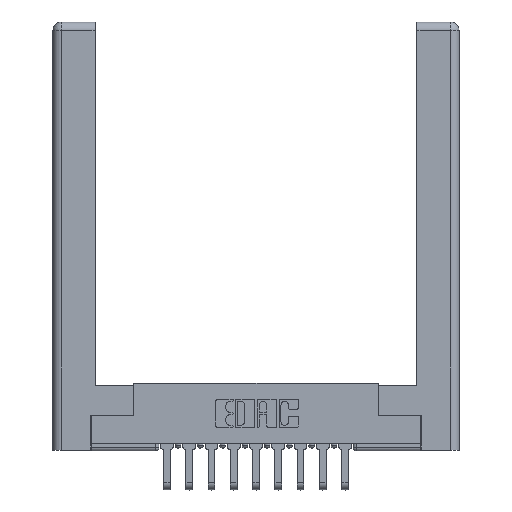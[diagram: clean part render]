
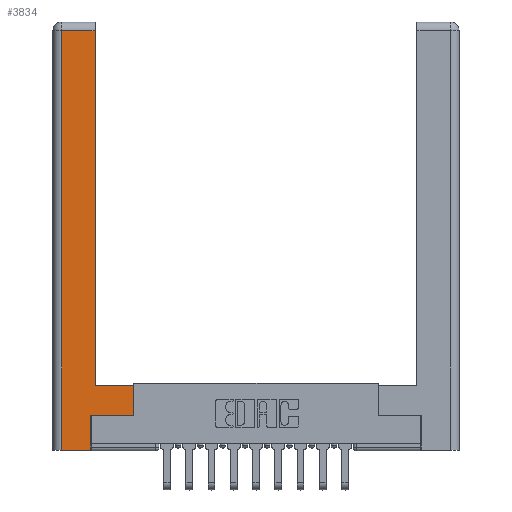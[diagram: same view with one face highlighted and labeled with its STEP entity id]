
A CAD part, top view. The second image highlights one B-rep face of the part: STEP entity #3834.
In plain terms, the highlighted planar face has unit normal (0, 0, 1).
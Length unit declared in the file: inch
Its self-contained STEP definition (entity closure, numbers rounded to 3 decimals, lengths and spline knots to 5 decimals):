
#125 = DIRECTION ( 'NONE',  ( 1., 0., 0. ) ) ;
#744 = CARTESIAN_POINT ( 'NONE',  ( 0.295, 2.94, 0. ) ) ;
#930 = VERTEX_POINT ( 'NONE', #9493 ) ;
#1247 = ORIENTED_EDGE ( 'NONE', *, *, #14229, .T. ) ;
#1302 = CARTESIAN_POINT ( 'NONE',  ( 0.565, 0.45, 0. ) ) ;
#1372 = DIRECTION ( 'NONE',  ( 0., 1., 0. ) ) ;
#1523 = EDGE_CURVE ( 'NONE', #11851, #3310, #7627, .T. ) ;
#1530 = VERTEX_POINT ( 'NONE', #10384 ) ;
#1573 = DIRECTION ( 'NONE',  ( -1., 0., 0. ) ) ;
#1775 = EDGE_CURVE ( 'NONE', #3623, #6599, #8016, .T. ) ;
#1843 = VECTOR ( 'NONE', #1372, 39.37008 ) ;
#1980 = CARTESIAN_POINT ( 'NONE',  ( 0.295, 0.45, 0. ) ) ;
#2111 = LINE ( 'NONE', #1980, #5832 ) ;
#2530 = VECTOR ( 'NONE', #13794, 39.37008 ) ;
#2933 = EDGE_CURVE ( 'NONE', #3310, #3623, #8172, .T. ) ;
#3310 = VERTEX_POINT ( 'NONE', #744 ) ;
#3444 = LINE ( 'NONE', #4160, #3625 ) ;
#3530 = ORIENTED_EDGE ( 'NONE', *, *, #1775, .T. ) ;
#3623 = VERTEX_POINT ( 'NONE', #16143 ) ;
#3625 = VECTOR ( 'NONE', #4552, 39.37008 ) ;
#3834 = ADVANCED_FACE ( 'NONE', ( #15181 ), #9052, .F. ) ;
#4160 = CARTESIAN_POINT ( 'NONE',  ( 0.265, 0., 0. ) ) ;
#4260 = DIRECTION ( 'NONE',  ( -1., 0., 0. ) ) ;
#4552 = DIRECTION ( 'NONE',  ( 1., 0., 0. ) ) ;
#4597 = CARTESIAN_POINT ( 'NONE',  ( 0.0615, 0., 0. ) ) ;
#4900 = LINE ( 'NONE', #6573, #11957 ) ;
#5036 = EDGE_CURVE ( 'NONE', #11642, #930, #8097, .T. ) ;
#5145 = AXIS2_PLACEMENT_3D ( 'NONE', #12853, #15372, #1573 ) ;
#5531 = ORIENTED_EDGE ( 'NONE', *, *, #15434, .T. ) ;
#5742 = VERTEX_POINT ( 'NONE', #1302 ) ;
#5832 = VECTOR ( 'NONE', #4260, 39.37008 ) ;
#6321 = CARTESIAN_POINT ( 'NONE',  ( 0.265, 0.245, 0. ) ) ;
#6382 = EDGE_LOOP ( 'NONE', ( #7853, #10713, #3530, #5531, #9889, #7190, #12267, #1247 ) ) ;
#6568 = CARTESIAN_POINT ( 'NONE',  ( 0.265, 0., 0. ) ) ;
#6573 = CARTESIAN_POINT ( 'NONE',  ( 0.565, 0.45, 0. ) ) ;
#6599 = VERTEX_POINT ( 'NONE', #4597 ) ;
#6864 = CARTESIAN_POINT ( 'NONE',  ( 0.0615, 2.94, 0. ) ) ;
#6979 = EDGE_CURVE ( 'NONE', #1530, #5742, #4900, .T. ) ;
#7190 = ORIENTED_EDGE ( 'NONE', *, *, #10307, .T. ) ;
#7627 = LINE ( 'NONE', #10085, #2530 ) ;
#7832 = DIRECTION ( 'NONE',  ( 0., 1., 0. ) ) ;
#7853 = ORIENTED_EDGE ( 'NONE', *, *, #1523, .T. ) ;
#8016 = LINE ( 'NONE', #11641, #13879 ) ;
#8097 = LINE ( 'NONE', #6321, #1843 ) ;
#8172 = LINE ( 'NONE', #6864, #13243 ) ;
#8491 = VECTOR ( 'NONE', #125, 39.37008 ) ;
#9052 = PLANE ( 'NONE',  #5145 ) ;
#9493 = CARTESIAN_POINT ( 'NONE',  ( 0.265, 0.245, 0. ) ) ;
#9889 = ORIENTED_EDGE ( 'NONE', *, *, #5036, .T. ) ;
#10085 = CARTESIAN_POINT ( 'NONE',  ( 0.295, 3., 0. ) ) ;
#10307 = EDGE_CURVE ( 'NONE', #930, #1530, #14760, .T. ) ;
#10384 = CARTESIAN_POINT ( 'NONE',  ( 0.565, 0.245, 0. ) ) ;
#10713 = ORIENTED_EDGE ( 'NONE', *, *, #2933, .T. ) ;
#11641 = CARTESIAN_POINT ( 'NONE',  ( 0.0615, 0., 0. ) ) ;
#11642 = VERTEX_POINT ( 'NONE', #6568 ) ;
#11851 = VERTEX_POINT ( 'NONE', #16055 ) ;
#11957 = VECTOR ( 'NONE', #7832, 39.37008 ) ;
#12267 = ORIENTED_EDGE ( 'NONE', *, *, #6979, .T. ) ;
#12483 = CARTESIAN_POINT ( 'NONE',  ( 0.565, 0.245, 0. ) ) ;
#12796 = DIRECTION ( 'NONE',  ( 0., -1., 0. ) ) ;
#12853 = CARTESIAN_POINT ( 'NONE',  ( 0., 0., 0. ) ) ;
#13243 = VECTOR ( 'NONE', #15487, 39.37008 ) ;
#13794 = DIRECTION ( 'NONE',  ( 0., 1., 0. ) ) ;
#13879 = VECTOR ( 'NONE', #12796, 39.37008 ) ;
#14229 = EDGE_CURVE ( 'NONE', #5742, #11851, #2111, .T. ) ;
#14760 = LINE ( 'NONE', #12483, #8491 ) ;
#15181 = FACE_OUTER_BOUND ( 'NONE', #6382, .T. ) ;
#15372 = DIRECTION ( 'NONE',  ( 0., 0., -1. ) ) ;
#15434 = EDGE_CURVE ( 'NONE', #6599, #11642, #3444, .T. ) ;
#15487 = DIRECTION ( 'NONE',  ( -1., 0., 0. ) ) ;
#16055 = CARTESIAN_POINT ( 'NONE',  ( 0.295, 0.45, 0. ) ) ;
#16143 = CARTESIAN_POINT ( 'NONE',  ( 0.0615, 2.94, 0. ) ) ;
